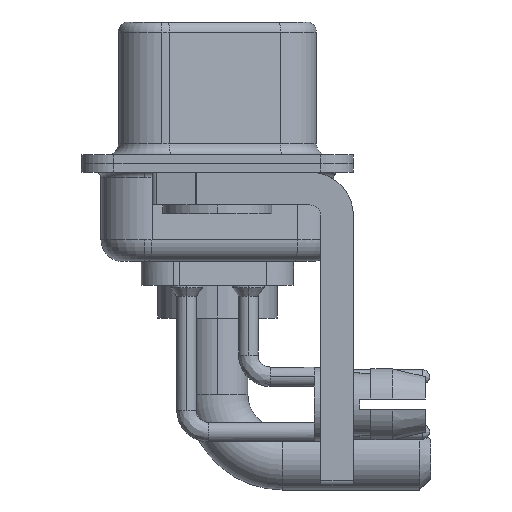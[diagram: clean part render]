
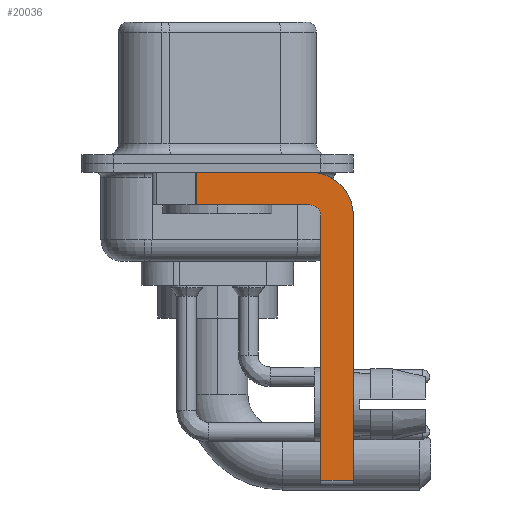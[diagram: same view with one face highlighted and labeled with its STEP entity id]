
A CAD part, left-side view. The second image highlights one B-rep face of the part: STEP entity #20036.
In plain terms, the highlighted planar face has unit normal (-1, 0, 0).
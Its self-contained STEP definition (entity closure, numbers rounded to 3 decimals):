
#200 = CARTESIAN_POINT ( 'NONE',  ( -2.9, -4.75, -14.8 ) ) ;
#549 = DIRECTION ( 'NONE',  ( 0., 0., -1. ) ) ;
#555 = VERTEX_POINT ( 'NONE', #15505 ) ;
#696 = LINE ( 'NONE', #10473, #5039 ) ;
#805 = VERTEX_POINT ( 'NONE', #9793 ) ;
#975 = VERTEX_POINT ( 'NONE', #20122 ) ;
#1017 = DIRECTION ( 'NONE',  ( -1., 0., 0. ) ) ;
#1037 = EDGE_CURVE ( 'NONE', #18713, #975, #17361, .T. ) ;
#1319 = EDGE_CURVE ( 'NONE', #4271, #555, #17008, .T. ) ;
#1502 = VECTOR ( 'NONE', #20204, 1000. ) ;
#1897 = ORIENTED_EDGE ( 'NONE', *, *, #16525, .T. ) ;
#2476 = CARTESIAN_POINT ( 'NONE',  ( -2.9, -4.75, -14.55 ) ) ;
#2644 = EDGE_CURVE ( 'NONE', #805, #4733, #20485, .T. ) ;
#2724 = VERTEX_POINT ( 'NONE', #2990 ) ;
#2990 = CARTESIAN_POINT ( 'NONE',  ( -2.9, -6.25, -14.55 ) ) ;
#3419 = EDGE_LOOP ( 'NONE', ( #3512, #1897, #18276, #11797, #5608, #10678, #20753, #5400 ) ) ;
#3512 = ORIENTED_EDGE ( 'NONE', *, *, #21025, .F. ) ;
#3526 = CARTESIAN_POINT ( 'NONE',  ( -2.9, -4.25, -2.4 ) ) ;
#3743 = DIRECTION ( 'NONE',  ( 1., 0., 0. ) ) ;
#3761 = CARTESIAN_POINT ( 'NONE',  ( -2.9, -4.25, -2.4 ) ) ;
#4271 = VERTEX_POINT ( 'NONE', #2476 ) ;
#4733 = VERTEX_POINT ( 'NONE', #19156 ) ;
#4888 = EDGE_CURVE ( 'NONE', #555, #18713, #8549, .T. ) ;
#5039 = VECTOR ( 'NONE', #17176, 1000. ) ;
#5400 = ORIENTED_EDGE ( 'NONE', *, *, #2644, .F. ) ;
#5590 = EDGE_CURVE ( 'NONE', #4733, #2724, #8627, .T. ) ;
#5608 = ORIENTED_EDGE ( 'NONE', *, *, #1319, .F. ) ;
#5945 = DIRECTION ( 'NONE',  ( 0., -1., 0. ) ) ;
#6801 = PLANE ( 'NONE',  #12028 ) ;
#6964 = CARTESIAN_POINT ( 'NONE',  ( -2.9, -6.25, -2.4 ) ) ;
#6999 = FACE_OUTER_BOUND ( 'NONE', #3419, .T. ) ;
#7270 = EDGE_CURVE ( 'NONE', #4271, #2724, #21114, .T. ) ;
#8549 = CIRCLE ( 'NONE', #20845, 0.5 ) ;
#8627 = LINE ( 'NONE', #6964, #10522 ) ;
#9013 = DIRECTION ( 'NONE',  ( 1., 0., 0. ) ) ;
#9793 = CARTESIAN_POINT ( 'NONE',  ( -2.9, -4.25, -0.4 ) ) ;
#9885 = CARTESIAN_POINT ( 'NONE',  ( -2.9, -4.25, -1.9 ) ) ;
#10473 = CARTESIAN_POINT ( 'NONE',  ( -2.9, 3., -0.4 ) ) ;
#10522 = VECTOR ( 'NONE', #10713, 1000. ) ;
#10649 = AXIS2_PLACEMENT_3D ( 'NONE', #3761, #9013, #549 ) ;
#10678 = ORIENTED_EDGE ( 'NONE', *, *, #7270, .T. ) ;
#10713 = DIRECTION ( 'NONE',  ( 0., 0., -1. ) ) ;
#11555 = CARTESIAN_POINT ( 'NONE',  ( -2.9, 0.978, -1.9 ) ) ;
#11797 = ORIENTED_EDGE ( 'NONE', *, *, #4888, .F. ) ;
#12028 = AXIS2_PLACEMENT_3D ( 'NONE', #3526, #3743, #13519 ) ;
#12881 = DIRECTION ( 'NONE',  ( 0., 0., 1. ) ) ;
#13212 = DIRECTION ( 'NONE',  ( 0., 0., -1. ) ) ;
#13347 = VECTOR ( 'NONE', #13212, 1000. ) ;
#13519 = DIRECTION ( 'NONE',  ( 0., 0., -1. ) ) ;
#14508 = CARTESIAN_POINT ( 'NONE',  ( -2.9, -4.25, -14.55 ) ) ;
#14516 = CARTESIAN_POINT ( 'NONE',  ( -2.9, -4.25, -2.4 ) ) ;
#14795 = CARTESIAN_POINT ( 'NONE',  ( -2.9, 0.978, -0.4 ) ) ;
#15505 = CARTESIAN_POINT ( 'NONE',  ( -2.9, -4.75, -2.4 ) ) ;
#15595 = CARTESIAN_POINT ( 'NONE',  ( -2.9, -4.25, -1.9 ) ) ;
#15698 = DIRECTION ( 'NONE',  ( 0., 1., 0. ) ) ;
#16525 = EDGE_CURVE ( 'NONE', #21698, #975, #20125, .T. ) ;
#17008 = LINE ( 'NONE', #200, #1502 ) ;
#17176 = DIRECTION ( 'NONE',  ( 0., -1., 0. ) ) ;
#17361 = LINE ( 'NONE', #15595, #20779 ) ;
#18276 = ORIENTED_EDGE ( 'NONE', *, *, #1037, .F. ) ;
#18713 = VERTEX_POINT ( 'NONE', #9885 ) ;
#19156 = CARTESIAN_POINT ( 'NONE',  ( -2.9, -6.25, -2.4 ) ) ;
#20025 = VECTOR ( 'NONE', #5945, 1000. ) ;
#20036 = ADVANCED_FACE ( 'NONE', ( #6999 ), #6801, .F. ) ;
#20122 = CARTESIAN_POINT ( 'NONE',  ( -2.9, 0.978, -1.9 ) ) ;
#20125 = LINE ( 'NONE', #11555, #13347 ) ;
#20204 = DIRECTION ( 'NONE',  ( 0., 0., 1. ) ) ;
#20485 = CIRCLE ( 'NONE', #10649, 2. ) ;
#20753 = ORIENTED_EDGE ( 'NONE', *, *, #5590, .F. ) ;
#20779 = VECTOR ( 'NONE', #15698, 1000. ) ;
#20845 = AXIS2_PLACEMENT_3D ( 'NONE', #14516, #1017, #12881 ) ;
#21025 = EDGE_CURVE ( 'NONE', #21698, #805, #696, .T. ) ;
#21114 = LINE ( 'NONE', #14508, #20025 ) ;
#21698 = VERTEX_POINT ( 'NONE', #14795 ) ;
